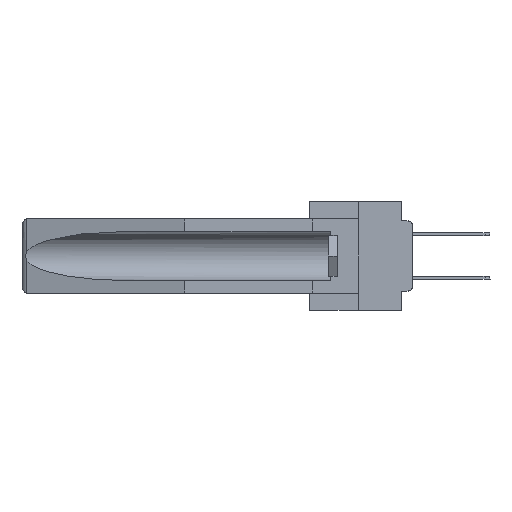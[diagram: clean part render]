
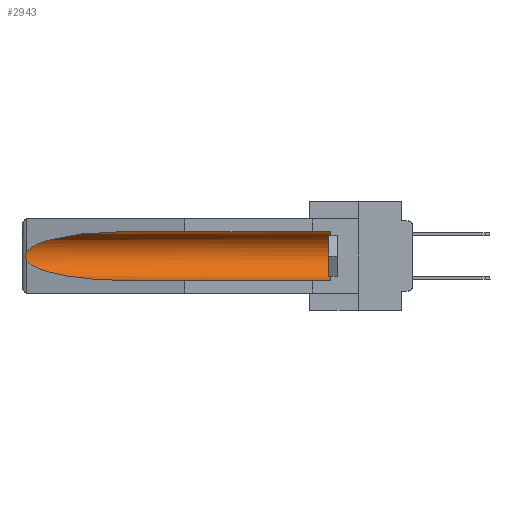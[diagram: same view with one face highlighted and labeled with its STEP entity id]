
A CAD part, left-side view. The second image highlights one B-rep face of the part: STEP entity #2943.
In plain terms, the highlighted cylindrical face has radius 2.857 mm (diameter 5.715 mm), a partial arc.
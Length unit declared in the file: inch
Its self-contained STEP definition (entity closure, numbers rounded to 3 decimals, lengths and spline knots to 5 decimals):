
#153 = CARTESIAN_POINT ( 'NONE',  ( 0.26537, 1.52718, -0.14972 ) ) ;
#372 = CARTESIAN_POINT ( 'NONE',  ( 0.26654, 1.53092, -0.15636 ) ) ;
#1275 = DIRECTION ( 'NONE',  ( 0., -1., 0. ) ) ;
#2484 = CARTESIAN_POINT ( 'NONE',  ( 0.26597, 1.5296, -0.19026 ) ) ;
#2774 = CARTESIAN_POINT ( 'NONE',  ( 0.155, 1.07973, -0.059 ) ) ;
#2943 = ADVANCED_FACE ( 'NONE', ( #30555 ), #24881, .F. ) ;
#3089 = ORIENTED_EDGE ( 'NONE', *, *, #7957, .F. ) ;
#3581 =( BOUNDED_CURVE ( )  B_SPLINE_CURVE ( 3, ( #8993, #21432, #23551, #4303 ),
 .UNSPECIFIED., .F., .T. ) 
 B_SPLINE_CURVE_WITH_KNOTS ( ( 4, 4 ),
 ( 4.71239, 6.08839 ),
 .UNSPECIFIED. ) 
 CURVE ( )  GEOMETRIC_REPRESENTATION_ITEM ( )  RATIONAL_B_SPLINE_CURVE ( ( 1., 0.848, 0.848, 1. ) ) 
 REPRESENTATION_ITEM ( '' )  );
#4303 = CARTESIAN_POINT ( 'NONE',  ( 0.26537, 1.52718, -0.14972 ) ) ;
#4822 = CARTESIAN_POINT ( 'NONE',  ( 0.2675, 1.53308, -0.17534 ) ) ;
#6155 = VERTEX_POINT ( 'NONE', #2774 ) ;
#7092 = CARTESIAN_POINT ( 'NONE',  ( 0.155, -0.30754, -0.1715 ) ) ;
#7111 = CARTESIAN_POINT ( 'NONE',  ( 0.155, 1.07973, -0.284 ) ) ;
#7327 = DIRECTION ( 'NONE',  ( 0., 1., 0. ) ) ;
#7481 = CARTESIAN_POINT ( 'NONE',  ( 0.26537, 1.52718, -0.19328 ) ) ;
#7822 = VERTEX_POINT ( 'NONE', #9135 ) ;
#7957 = EDGE_CURVE ( 'NONE', #19532, #8226, #16487, .T. ) ;
#7968 = CARTESIAN_POINT ( 'NONE',  ( 0.26537, 1.52718, -0.19328 ) ) ;
#8226 = VERTEX_POINT ( 'NONE', #10776 ) ;
#8807 = AXIS2_PLACEMENT_3D ( 'NONE', #7092, #23963, #21644 ) ;
#8993 = CARTESIAN_POINT ( 'NONE',  ( 0.155, 1.07973, -0.059 ) ) ;
#9135 = CARTESIAN_POINT ( 'NONE',  ( 0.26537, 1.52718, -0.14972 ) ) ;
#9149 = ORIENTED_EDGE ( 'NONE', *, *, #9577, .T. ) ;
#9577 = EDGE_CURVE ( 'NONE', #10778, #8226, #21007, .T. ) ;
#9642 = CARTESIAN_POINT ( 'NONE',  ( 0.21114, 1.30732, -0.284 ) ) ;
#10776 = CARTESIAN_POINT ( 'NONE',  ( 0.155, 1.07973, -0.284 ) ) ;
#10778 = VERTEX_POINT ( 'NONE', #7968 ) ;
#11142 = B_SPLINE_CURVE_WITH_KNOTS ( 'NONE', 3,
 ( #153, #28949, #372, #14872, #17295, #4822, #19518, #17093, #2484, #7481 ),
 .UNSPECIFIED., .F., .F.,
 ( 4, 2, 2, 2, 4 ),
 ( 0., 0.00029, 0.00058, 0.00087, 0.00117 ),
 .UNSPECIFIED. ) ;
#11670 = CIRCLE ( 'NONE', #22262, 0.1125 ) ;
#11963 = CARTESIAN_POINT ( 'NONE',  ( 0.155, -0.30754, -0.284 ) ) ;
#12439 = CARTESIAN_POINT ( 'NONE',  ( 0.155, 0.126, -0.059 ) ) ;
#12526 = EDGE_CURVE ( 'NONE', #22598, #6155, #15848, .T. ) ;
#13785 = ORIENTED_EDGE ( 'NONE', *, *, #21814, .T. ) ;
#14623 = DIRECTION ( 'NONE',  ( 0., 1., 0. ) ) ;
#14872 = CARTESIAN_POINT ( 'NONE',  ( 0.2673, 1.5327, -0.16383 ) ) ;
#15848 = LINE ( 'NONE', #21894, #23004 ) ;
#16487 = LINE ( 'NONE', #11963, #27067 ) ;
#16819 = CARTESIAN_POINT ( 'NONE',  ( 0.25451, 1.48313, -0.24835 ) ) ;
#17093 = CARTESIAN_POINT ( 'NONE',  ( 0.26655, 1.53094, -0.18657 ) ) ;
#17295 = CARTESIAN_POINT ( 'NONE',  ( 0.2675, 1.53308, -0.16763 ) ) ;
#17647 = EDGE_CURVE ( 'NONE', #7822, #10778, #11142, .T. ) ;
#18398 = CARTESIAN_POINT ( 'NONE',  ( 0.155, 0.126, -0.1715 ) ) ;
#19518 = CARTESIAN_POINT ( 'NONE',  ( 0.2673, 1.53269, -0.17917 ) ) ;
#19532 = VERTEX_POINT ( 'NONE', #24121 ) ;
#20013 = EDGE_LOOP ( 'NONE', ( #28645, #30419, #9149, #3089, #13785, #21951 ) ) ;
#21007 =( BOUNDED_CURVE ( )  B_SPLINE_CURVE ( 3, ( #28558, #16819, #9642, #7111 ),
 .UNSPECIFIED., .F., .F. ) 
 B_SPLINE_CURVE_WITH_KNOTS ( ( 4, 4 ),
 ( 0.1948, 1.5708 ),
 .UNSPECIFIED. ) 
 CURVE ( )  GEOMETRIC_REPRESENTATION_ITEM ( )  RATIONAL_B_SPLINE_CURVE ( ( 1., 0.848, 0.848, 1. ) ) 
 REPRESENTATION_ITEM ( '' )  );
#21432 = CARTESIAN_POINT ( 'NONE',  ( 0.21114, 1.30732, -0.059 ) ) ;
#21644 = DIRECTION ( 'NONE',  ( 0., 0., 1. ) ) ;
#21814 = EDGE_CURVE ( 'NONE', #19532, #22598, #11670, .T. ) ;
#21894 = CARTESIAN_POINT ( 'NONE',  ( 0.155, -0.30754, -0.059 ) ) ;
#21951 = ORIENTED_EDGE ( 'NONE', *, *, #12526, .T. ) ;
#22262 = AXIS2_PLACEMENT_3D ( 'NONE', #18398, #1275, #28147 ) ;
#22598 = VERTEX_POINT ( 'NONE', #12439 ) ;
#23004 = VECTOR ( 'NONE', #14623, 39.37008 ) ;
#23551 = CARTESIAN_POINT ( 'NONE',  ( 0.25451, 1.48313, -0.09465 ) ) ;
#23963 = DIRECTION ( 'NONE',  ( 0., 1., 0. ) ) ;
#24121 = CARTESIAN_POINT ( 'NONE',  ( 0.155, 0.126, -0.284 ) ) ;
#24319 = EDGE_CURVE ( 'NONE', #6155, #7822, #3581, .T. ) ;
#24881 = CYLINDRICAL_SURFACE ( 'NONE', #8807, 0.1125 ) ;
#27067 = VECTOR ( 'NONE', #7327, 39.37008 ) ;
#28147 = DIRECTION ( 'NONE',  ( 0., 0., 1. ) ) ;
#28558 = CARTESIAN_POINT ( 'NONE',  ( 0.26537, 1.52718, -0.19328 ) ) ;
#28645 = ORIENTED_EDGE ( 'NONE', *, *, #24319, .T. ) ;
#28949 = CARTESIAN_POINT ( 'NONE',  ( 0.26597, 1.52961, -0.15275 ) ) ;
#30419 = ORIENTED_EDGE ( 'NONE', *, *, #17647, .T. ) ;
#30555 = FACE_OUTER_BOUND ( 'NONE', #20013, .T. ) ;
